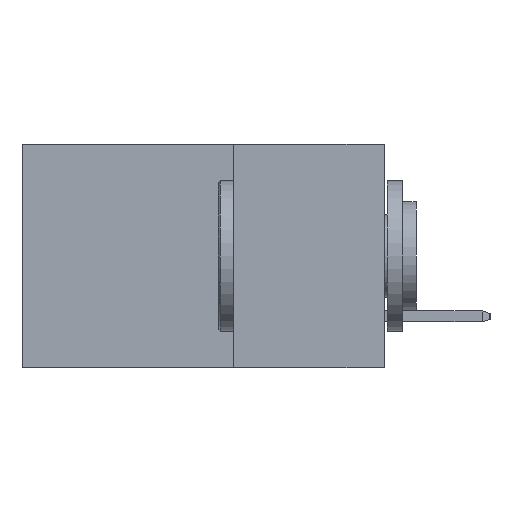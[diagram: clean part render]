
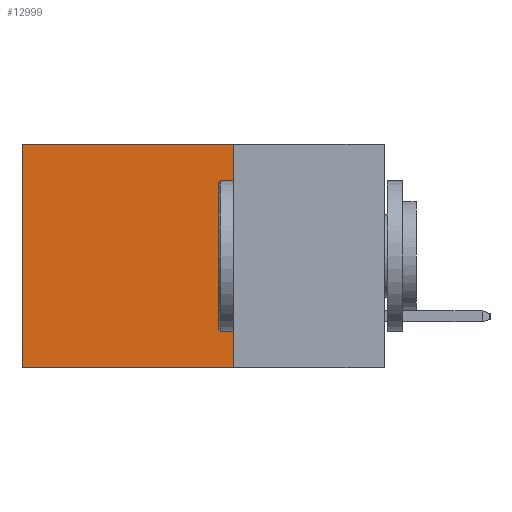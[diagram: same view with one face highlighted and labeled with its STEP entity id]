
A CAD part, left-side view. The second image highlights one B-rep face of the part: STEP entity #12999.
In plain terms, the highlighted planar face has unit normal (-1, 0, 0).
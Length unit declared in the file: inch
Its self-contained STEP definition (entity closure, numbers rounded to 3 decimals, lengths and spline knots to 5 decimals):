
#819 = CARTESIAN_POINT ( 'NONE',  ( 0.298, 0.6, -0.37 ) ) ;
#851 = FACE_OUTER_BOUND ( 'NONE', #5252, .T. ) ;
#1655 = CARTESIAN_POINT ( 'NONE',  ( 0.298, 0.6, 0. ) ) ;
#2725 = EDGE_CURVE ( 'NONE', #14621, #16357, #18966, .T. ) ;
#2770 = VECTOR ( 'NONE', #18780, 39.37008 ) ;
#3864 = EDGE_CURVE ( 'NONE', #17713, #4940, #6872, .T. ) ;
#4389 = DIRECTION ( 'NONE',  ( 0., 1., 0. ) ) ;
#4940 = VERTEX_POINT ( 'NONE', #14376 ) ;
#5252 = EDGE_LOOP ( 'NONE', ( #14305, #10874, #6874, #7510 ) ) ;
#5456 = CARTESIAN_POINT ( 'NONE',  ( 0.298, 0.25, 0. ) ) ;
#6872 = LINE ( 'NONE', #15993, #2770 ) ;
#6874 = ORIENTED_EDGE ( 'NONE', *, *, #3864, .F. ) ;
#7510 = ORIENTED_EDGE ( 'NONE', *, *, #13800, .T. ) ;
#7762 = DIRECTION ( 'NONE',  ( 0., 0., -1. ) ) ;
#8550 = DIRECTION ( 'NONE',  ( 1., 0., 0. ) ) ;
#9603 = CARTESIAN_POINT ( 'NONE',  ( 0.298, 0.25, -0.37 ) ) ;
#9694 = AXIS2_PLACEMENT_3D ( 'NONE', #5456, #8550, #18452 ) ;
#10874 = ORIENTED_EDGE ( 'NONE', *, *, #13455, .F. ) ;
#11564 = LINE ( 'NONE', #9603, #14864 ) ;
#12025 = VECTOR ( 'NONE', #4389, 39.37008 ) ;
#12999 = ADVANCED_FACE ( 'NONE', ( #851 ), #17030, .F. ) ;
#13336 = CARTESIAN_POINT ( 'NONE',  ( 0.298, 0.25, 0. ) ) ;
#13455 = EDGE_CURVE ( 'NONE', #4940, #16357, #11564, .T. ) ;
#13606 = CARTESIAN_POINT ( 'NONE',  ( 0.298, 0.6, 0. ) ) ;
#13800 = EDGE_CURVE ( 'NONE', #17713, #14621, #16107, .T. ) ;
#14305 = ORIENTED_EDGE ( 'NONE', *, *, #2725, .T. ) ;
#14376 = CARTESIAN_POINT ( 'NONE',  ( 0.298, 0.25, -0.37 ) ) ;
#14592 = CARTESIAN_POINT ( 'NONE',  ( 0.298, 0.25, 0. ) ) ;
#14621 = VERTEX_POINT ( 'NONE', #13606 ) ;
#14864 = VECTOR ( 'NONE', #16619, 39.37008 ) ;
#15993 = CARTESIAN_POINT ( 'NONE',  ( 0.298, 0.25, 0. ) ) ;
#16107 = LINE ( 'NONE', #13336, #12025 ) ;
#16357 = VERTEX_POINT ( 'NONE', #819 ) ;
#16619 = DIRECTION ( 'NONE',  ( 0., 1., 0. ) ) ;
#17030 = PLANE ( 'NONE',  #9694 ) ;
#17713 = VERTEX_POINT ( 'NONE', #14592 ) ;
#18452 = DIRECTION ( 'NONE',  ( 0., 0., -1. ) ) ;
#18514 = VECTOR ( 'NONE', #7762, 39.37008 ) ;
#18780 = DIRECTION ( 'NONE',  ( 0., 0., -1. ) ) ;
#18966 = LINE ( 'NONE', #1655, #18514 ) ;
